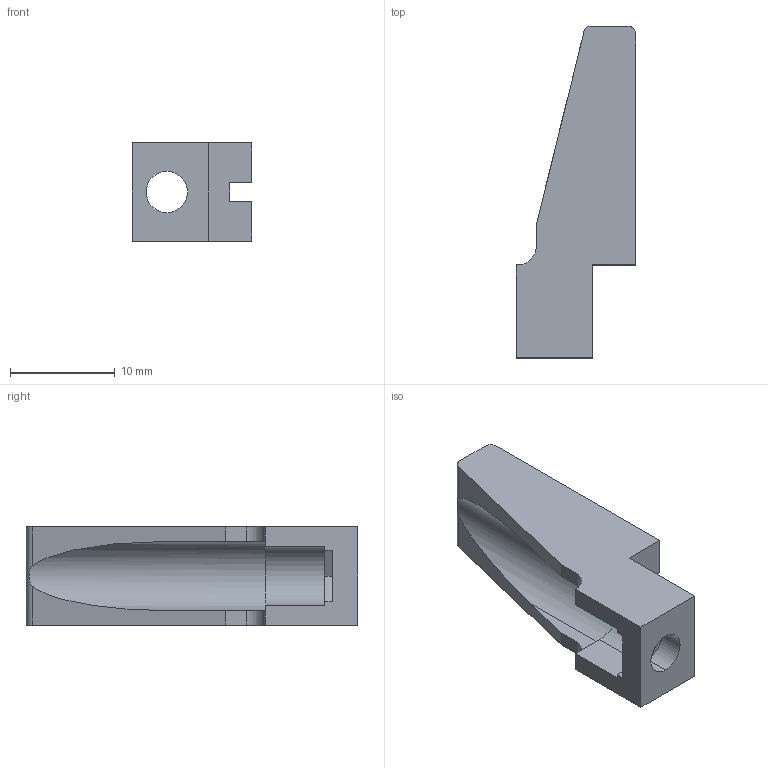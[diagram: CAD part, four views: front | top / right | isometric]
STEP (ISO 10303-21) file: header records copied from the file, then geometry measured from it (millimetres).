
FILE_DESCRIPTION (( 'STEP AP214' ), '1' );
FILE_NAME ('345-220-088.STEP', '2020-08-18T19:19:29', ( '' ), ( '' ), 'SwSTEP 2.0', 'SolidWorks 2020', '' );
FILE_SCHEMA (( 'AUTOMOTIVE_DESIGN' ));
Length unit declared in the file: inch
Products named in the file (1): 345-220-088
Bounding box: 11.44 x 31.75 x 9.4 mm (x, y, z)
Volume: 1593.1 mm3; surface area: 1497.6 mm2
Topology: 1 solids, 1 shells, 39 faces, 107 edges, 70 vertices
Faces by surface type: plane 27, cylinder 12
Entity records: 1292 total; most frequent: CARTESIAN_POINT 248, ORIENTED_EDGE 214, DIRECTION 195, EDGE_CURVE 107, VECTOR 85, LINE 85, VERTEX_POINT 70, AXIS2_PLACEMENT_3D 55
